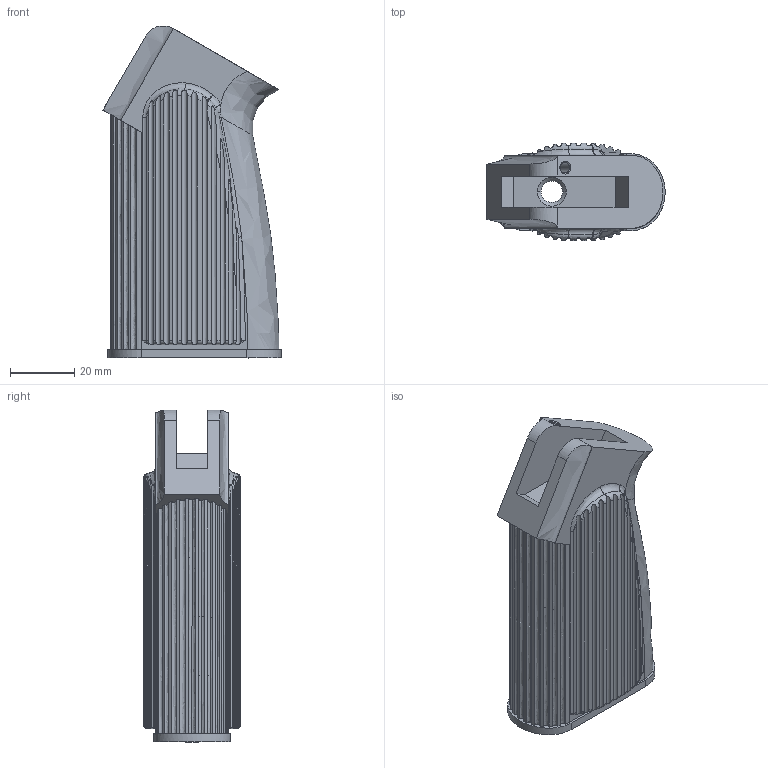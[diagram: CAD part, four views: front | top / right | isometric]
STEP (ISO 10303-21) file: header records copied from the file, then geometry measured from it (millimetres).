
FILE_DESCRIPTION (( 'STEP AP203' ), '1' );
FILE_NAME ('AF-WF-PG-PRT-001-STEP.STEP', '2020-07-21T23:59:15', ( '' ), ( '' ), 'SwSTEP 2.0', 'SolidWorks 2018', '' );
FILE_SCHEMA (( 'CONFIG_CONTROL_DESIGN' ));
Length unit declared in the file: inch
Products named in the file (1): AF-WF-PG-PRT-001-STEP
Bounding box: 55.64 x 30.43 x 103.74 mm (x, y, z)
Volume: 60178.8 mm3; surface area: 25146.4 mm2
Topology: 1 solids, 1 shells, 191 faces, 517 edges, 331 vertices
Faces by surface type: bspline 68, cylinder 66, plane 35, cone 12, torus 10
Entity records: 9209 total; most frequent: CARTESIAN_POINT 5005, ORIENTED_EDGE 1034, DIRECTION 639, EDGE_CURVE 517, VERTEX_POINT 331, AXIS2_PLACEMENT_3D 234, B_SPLINE_CURVE_WITH_KNOTS 205, EDGE_LOOP 196
